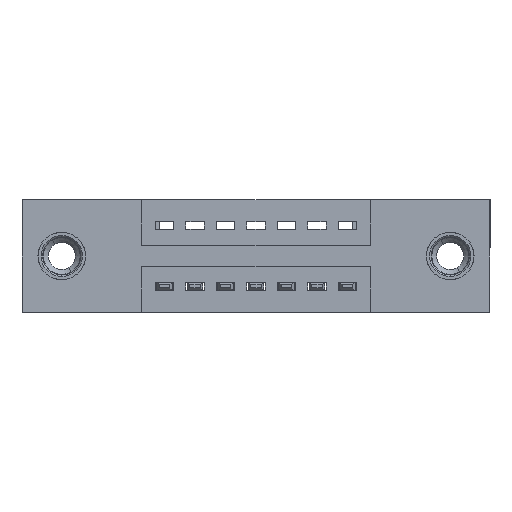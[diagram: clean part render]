
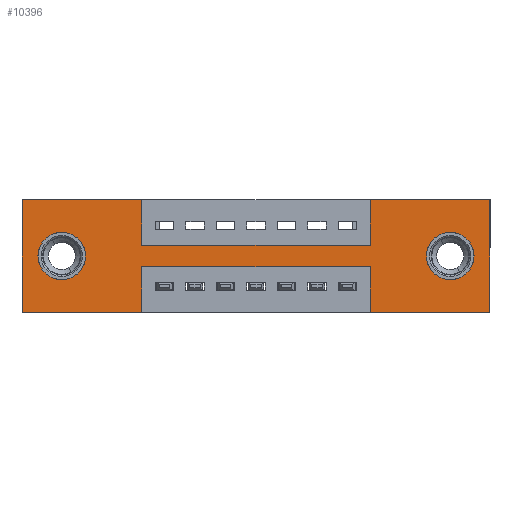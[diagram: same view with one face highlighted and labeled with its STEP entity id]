
A CAD part, front view. The second image highlights one B-rep face of the part: STEP entity #10396.
In plain terms, the highlighted planar face has unit normal (0, -1, 0).
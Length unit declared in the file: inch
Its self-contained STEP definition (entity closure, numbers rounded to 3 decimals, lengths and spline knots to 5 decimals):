
#6 = EDGE_LOOP ( 'NONE', ( #8264, #8440, #4699, #4803, #3527, #4895, #11152, #348, #8595, #6136, #11724, #6391 ) ) ;
#15 = EDGE_CURVE ( 'NONE', #4223, #1744, #1196, .T. ) ;
#50 = DIRECTION ( 'NONE',  ( 1., 0., 0. ) ) ;
#67 = EDGE_LOOP ( 'NONE', ( #3264, #7838 ) ) ;
#215 = VERTEX_POINT ( 'NONE', #8116 ) ;
#245 = DIRECTION ( 'NONE',  ( 0., 0., -1. ) ) ;
#348 = ORIENTED_EDGE ( 'NONE', *, *, #15, .F. ) ;
#533 = EDGE_CURVE ( 'NONE', #3490, #5361, #2805, .T. ) ;
#590 = VECTOR ( 'NONE', #4204, 39.37008 ) ;
#661 = CARTESIAN_POINT ( 'NONE',  ( 0.13, 0., -0.263 ) ) ;
#759 = DIRECTION ( 'NONE',  ( -1., 0., 0. ) ) ;
#801 = CARTESIAN_POINT ( 'NONE',  ( 0., 0., -0.37 ) ) ;
#833 = DIRECTION ( 'NONE',  ( 0., 0., 1. ) ) ;
#847 = DIRECTION ( 'NONE',  ( -1., 0., 0. ) ) ;
#1029 = EDGE_CURVE ( 'NONE', #3794, #8947, #1760, .T. ) ;
#1112 = DIRECTION ( 'NONE',  ( 1., 0., 0. ) ) ;
#1196 = LINE ( 'NONE', #11238, #9711 ) ;
#1323 = CARTESIAN_POINT ( 'NONE',  ( 0., 0., -0.37 ) ) ;
#1396 = VERTEX_POINT ( 'NONE', #8492 ) ;
#1516 = EDGE_CURVE ( 'NONE', #4926, #10546, #8395, .T. ) ;
#1744 = VERTEX_POINT ( 'NONE', #11901 ) ;
#1755 = LINE ( 'NONE', #7841, #4076 ) ;
#1760 = LINE ( 'NONE', #11606, #4081 ) ;
#2036 = VERTEX_POINT ( 'NONE', #5571 ) ;
#2149 = ORIENTED_EDGE ( 'NONE', *, *, #2372, .T. ) ;
#2158 = VECTOR ( 'NONE', #833, 39.37008 ) ;
#2178 = FACE_OUTER_BOUND ( 'NONE', #6, .T. ) ;
#2372 = EDGE_CURVE ( 'NONE', #11715, #215, #9386, .T. ) ;
#2549 = CARTESIAN_POINT ( 'NONE',  ( 1.535, 0., 0. ) ) ;
#2573 = EDGE_CURVE ( 'NONE', #1396, #4128, #9518, .T. ) ;
#2805 = CIRCLE ( 'NONE', #11875, 0.078 ) ;
#2870 = CARTESIAN_POINT ( 'NONE',  ( 0., 0., 0. ) ) ;
#3048 = CARTESIAN_POINT ( 'NONE',  ( 0.3925, 0., 0. ) ) ;
#3264 = ORIENTED_EDGE ( 'NONE', *, *, #6560, .T. ) ;
#3475 = DIRECTION ( 'NONE',  ( 0., 0., 1. ) ) ;
#3476 = FACE_BOUND ( 'NONE', #67, .T. ) ;
#3490 = VERTEX_POINT ( 'NONE', #661 ) ;
#3515 = CARTESIAN_POINT ( 'NONE',  ( 1.1425, 0., 0. ) ) ;
#3527 = ORIENTED_EDGE ( 'NONE', *, *, #9597, .F. ) ;
#3591 = CARTESIAN_POINT ( 'NONE',  ( 1.405, 0., -0.185 ) ) ;
#3764 = CARTESIAN_POINT ( 'NONE',  ( 0.3925, 0., -0.15 ) ) ;
#3794 = VERTEX_POINT ( 'NONE', #5112 ) ;
#3848 = CARTESIAN_POINT ( 'NONE',  ( 0.13, 0., -0.107 ) ) ;
#3967 = CARTESIAN_POINT ( 'NONE',  ( 0., 0., 0. ) ) ;
#4076 = VECTOR ( 'NONE', #10617, 39.37008 ) ;
#4081 = VECTOR ( 'NONE', #9791, 39.37008 ) ;
#4126 = CARTESIAN_POINT ( 'NONE',  ( 1.1425, 0., -0.37 ) ) ;
#4128 = VERTEX_POINT ( 'NONE', #5890 ) ;
#4204 = DIRECTION ( 'NONE',  ( 0., 0., 1. ) ) ;
#4223 = VERTEX_POINT ( 'NONE', #3764 ) ;
#4288 = VERTEX_POINT ( 'NONE', #2549 ) ;
#4344 = CARTESIAN_POINT ( 'NONE',  ( 1.1425, 0., -0.22 ) ) ;
#4376 = EDGE_CURVE ( 'NONE', #215, #11715, #6719, .T. ) ;
#4428 = CARTESIAN_POINT ( 'NONE',  ( 0.13, 0., -0.185 ) ) ;
#4598 = EDGE_CURVE ( 'NONE', #8947, #1396, #5439, .T. ) ;
#4699 = ORIENTED_EDGE ( 'NONE', *, *, #1516, .F. ) ;
#4803 = ORIENTED_EDGE ( 'NONE', *, *, #5105, .F. ) ;
#4895 = ORIENTED_EDGE ( 'NONE', *, *, #10883, .F. ) ;
#4926 = VERTEX_POINT ( 'NONE', #7507 ) ;
#5105 = EDGE_CURVE ( 'NONE', #11878, #4926, #6138, .T. ) ;
#5112 = CARTESIAN_POINT ( 'NONE',  ( 0.3925, 0., -0.22 ) ) ;
#5361 = VERTEX_POINT ( 'NONE', #3848 ) ;
#5439 = LINE ( 'NONE', #801, #10763 ) ;
#5441 = LINE ( 'NONE', #7147, #8334 ) ;
#5517 = DIRECTION ( 'NONE',  ( 0., 1., 0. ) ) ;
#5571 = CARTESIAN_POINT ( 'NONE',  ( 1.1425, 0., 0. ) ) ;
#5673 = ORIENTED_EDGE ( 'NONE', *, *, #4376, .T. ) ;
#5701 = VECTOR ( 'NONE', #10415, 39.37008 ) ;
#5890 = CARTESIAN_POINT ( 'NONE',  ( 0., 0., 0. ) ) ;
#5911 = VECTOR ( 'NONE', #1112, 39.37008 ) ;
#6136 = ORIENTED_EDGE ( 'NONE', *, *, #10893, .F. ) ;
#6138 = LINE ( 'NONE', #11910, #10323 ) ;
#6203 = EDGE_CURVE ( 'NONE', #10546, #3794, #5441, .T. ) ;
#6391 = ORIENTED_EDGE ( 'NONE', *, *, #4598, .F. ) ;
#6560 = EDGE_CURVE ( 'NONE', #5361, #3490, #11648, .T. ) ;
#6719 = CIRCLE ( 'NONE', #11228, 0.078 ) ;
#6769 = FACE_BOUND ( 'NONE', #7280, .T. ) ;
#6772 = LINE ( 'NONE', #3967, #5911 ) ;
#6872 = CARTESIAN_POINT ( 'NONE',  ( 0.13, 0., -0.185 ) ) ;
#6950 = AXIS2_PLACEMENT_3D ( 'NONE', #1323, #10365, #245 ) ;
#7147 = CARTESIAN_POINT ( 'NONE',  ( 0.3925, 0., -0.22 ) ) ;
#7280 = EDGE_LOOP ( 'NONE', ( #2149, #5673 ) ) ;
#7402 = EDGE_CURVE ( 'NONE', #11817, #4223, #9173, .T. ) ;
#7507 = CARTESIAN_POINT ( 'NONE',  ( 1.1425, 0., -0.37 ) ) ;
#7615 = AXIS2_PLACEMENT_3D ( 'NONE', #3591, #5517, #11945 ) ;
#7838 = ORIENTED_EDGE ( 'NONE', *, *, #533, .T. ) ;
#7841 = CARTESIAN_POINT ( 'NONE',  ( 1.535, 0., 0. ) ) ;
#8101 = DIRECTION ( 'NONE',  ( 0., 1., 0. ) ) ;
#8116 = CARTESIAN_POINT ( 'NONE',  ( 1.405, 0., -0.263 ) ) ;
#8235 = CARTESIAN_POINT ( 'NONE',  ( 0.3925, 0., 0. ) ) ;
#8264 = ORIENTED_EDGE ( 'NONE', *, *, #1029, .F. ) ;
#8334 = VECTOR ( 'NONE', #11811, 39.37008 ) ;
#8365 = VECTOR ( 'NONE', #11830, 39.37008 ) ;
#8395 = LINE ( 'NONE', #4126, #590 ) ;
#8440 = ORIENTED_EDGE ( 'NONE', *, *, #6203, .F. ) ;
#8460 = DIRECTION ( 'NONE',  ( 1., 0., 0. ) ) ;
#8492 = CARTESIAN_POINT ( 'NONE',  ( 0., 0., -0.37 ) ) ;
#8595 = ORIENTED_EDGE ( 'NONE', *, *, #7402, .F. ) ;
#8854 = DIRECTION ( 'NONE',  ( 0., 0., 1. ) ) ;
#8936 = LINE ( 'NONE', #3515, #8365 ) ;
#8947 = VERTEX_POINT ( 'NONE', #10871 ) ;
#9173 = LINE ( 'NONE', #3048, #5701 ) ;
#9386 = CIRCLE ( 'NONE', #7615, 0.078 ) ;
#9451 = PLANE ( 'NONE',  #6950 ) ;
#9518 = LINE ( 'NONE', #10012, #2158 ) ;
#9597 = EDGE_CURVE ( 'NONE', #4288, #11878, #1755, .T. ) ;
#9711 = VECTOR ( 'NONE', #50, 39.37008 ) ;
#9778 = DIRECTION ( 'NONE',  ( 0., 1., 0. ) ) ;
#9791 = DIRECTION ( 'NONE',  ( 0., 0., -1. ) ) ;
#9849 = CARTESIAN_POINT ( 'NONE',  ( 1.405, 0., -0.185 ) ) ;
#10012 = CARTESIAN_POINT ( 'NONE',  ( 0., 0., 0. ) ) ;
#10323 = VECTOR ( 'NONE', #847, 39.37008 ) ;
#10365 = DIRECTION ( 'NONE',  ( 0., -1., 0. ) ) ;
#10396 = ADVANCED_FACE ( 'NONE', ( #6769, #3476, #2178 ), #9451, .T. ) ;
#10415 = DIRECTION ( 'NONE',  ( 0., 0., -1. ) ) ;
#10546 = VERTEX_POINT ( 'NONE', #4344 ) ;
#10576 = EDGE_CURVE ( 'NONE', #1744, #2036, #8936, .T. ) ;
#10610 = DIRECTION ( 'NONE',  ( 0., 1., 0. ) ) ;
#10617 = DIRECTION ( 'NONE',  ( 0., 0., -1. ) ) ;
#10763 = VECTOR ( 'NONE', #759, 39.37008 ) ;
#10769 = CARTESIAN_POINT ( 'NONE',  ( 1.405, 0., -0.107 ) ) ;
#10796 = AXIS2_PLACEMENT_3D ( 'NONE', #4428, #8101, #3475 ) ;
#10871 = CARTESIAN_POINT ( 'NONE',  ( 0.3925, 0., -0.37 ) ) ;
#10883 = EDGE_CURVE ( 'NONE', #2036, #4288, #6772, .T. ) ;
#10893 = EDGE_CURVE ( 'NONE', #4128, #11817, #11544, .T. ) ;
#10895 = CARTESIAN_POINT ( 'NONE',  ( 1.535, 0., -0.37 ) ) ;
#11152 = ORIENTED_EDGE ( 'NONE', *, *, #10576, .F. ) ;
#11228 = AXIS2_PLACEMENT_3D ( 'NONE', #9849, #10610, #11547 ) ;
#11238 = CARTESIAN_POINT ( 'NONE',  ( 0.3925, 0., -0.15 ) ) ;
#11270 = VECTOR ( 'NONE', #8460, 39.37008 ) ;
#11544 = LINE ( 'NONE', #2870, #11270 ) ;
#11547 = DIRECTION ( 'NONE',  ( 0., 0., -1. ) ) ;
#11606 = CARTESIAN_POINT ( 'NONE',  ( 0.3925, 0., -0.37 ) ) ;
#11648 = CIRCLE ( 'NONE', #10796, 0.078 ) ;
#11715 = VERTEX_POINT ( 'NONE', #10769 ) ;
#11724 = ORIENTED_EDGE ( 'NONE', *, *, #2573, .F. ) ;
#11811 = DIRECTION ( 'NONE',  ( -1., 0., 0. ) ) ;
#11817 = VERTEX_POINT ( 'NONE', #8235 ) ;
#11830 = DIRECTION ( 'NONE',  ( 0., 0., 1. ) ) ;
#11875 = AXIS2_PLACEMENT_3D ( 'NONE', #6872, #9778, #8854 ) ;
#11878 = VERTEX_POINT ( 'NONE', #10895 ) ;
#11901 = CARTESIAN_POINT ( 'NONE',  ( 1.1425, 0., -0.15 ) ) ;
#11910 = CARTESIAN_POINT ( 'NONE',  ( 0., 0., -0.37 ) ) ;
#11945 = DIRECTION ( 'NONE',  ( 0., 0., -1. ) ) ;
